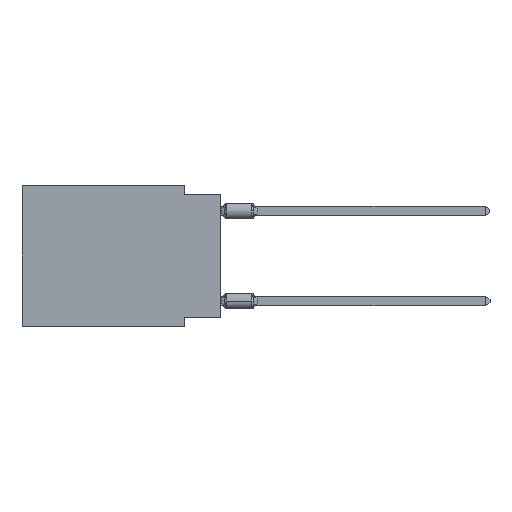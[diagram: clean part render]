
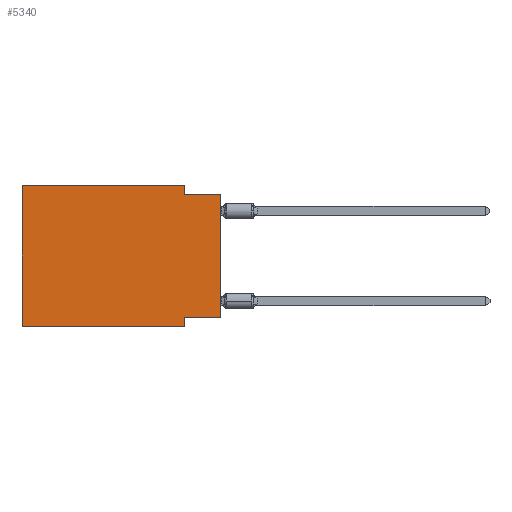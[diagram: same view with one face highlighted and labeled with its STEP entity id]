
A CAD part, left-side view. The second image highlights one B-rep face of the part: STEP entity #5340.
In plain terms, the highlighted planar face has unit normal (-1, 0, 0).
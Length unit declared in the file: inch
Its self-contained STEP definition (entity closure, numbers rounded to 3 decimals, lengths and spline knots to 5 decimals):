
#259 = LINE ( 'NONE', #17648, #6496 ) ;
#445 = EDGE_CURVE ( 'NONE', #4092, #9100, #18536, .T. ) ;
#514 = VERTEX_POINT ( 'NONE', #1994 ) ;
#1445 = EDGE_LOOP ( 'NONE', ( #12700, #13799, #5948, #2349, #14750, #10892, #8039, #2015 ) ) ;
#1649 = CARTESIAN_POINT ( 'NONE',  ( 0., 0.1, -0.025 ) ) ;
#1694 = VECTOR ( 'NONE', #16999, 39.37008 ) ;
#1905 = CARTESIAN_POINT ( 'NONE',  ( 0., 0., -0.365 ) ) ;
#1994 = CARTESIAN_POINT ( 'NONE',  ( 0., 0.1, 0. ) ) ;
#2015 = ORIENTED_EDGE ( 'NONE', *, *, #4276, .F. ) ;
#2109 = CARTESIAN_POINT ( 'NONE',  ( 0., 0.55, -0.39 ) ) ;
#2139 = CARTESIAN_POINT ( 'NONE',  ( 0., 0.55, 0. ) ) ;
#2317 = CARTESIAN_POINT ( 'NONE',  ( 0., 0.55, 0. ) ) ;
#2349 = ORIENTED_EDGE ( 'NONE', *, *, #6846, .F. ) ;
#2357 = CARTESIAN_POINT ( 'NONE',  ( 0., 0.1, -0.365 ) ) ;
#2386 = EDGE_CURVE ( 'NONE', #9490, #3040, #17271, .T. ) ;
#2815 = CARTESIAN_POINT ( 'NONE',  ( 0., 0.55, 0. ) ) ;
#2879 = VECTOR ( 'NONE', #5657, 39.37008 ) ;
#3040 = VERTEX_POINT ( 'NONE', #16275 ) ;
#3069 = DIRECTION ( 'NONE',  ( 0., 0., 1. ) ) ;
#3242 = VECTOR ( 'NONE', #17479, 39.37008 ) ;
#3299 = EDGE_CURVE ( 'NONE', #15365, #9100, #11369, .T. ) ;
#3946 = VERTEX_POINT ( 'NONE', #2317 ) ;
#4092 = VERTEX_POINT ( 'NONE', #18384 ) ;
#4115 = AXIS2_PLACEMENT_3D ( 'NONE', #2139, #12278, #6644 ) ;
#4240 = CARTESIAN_POINT ( 'NONE',  ( 0., 0., -0.025 ) ) ;
#4276 = EDGE_CURVE ( 'NONE', #4092, #9490, #10543, .T. ) ;
#5052 = VECTOR ( 'NONE', #8529, 39.37008 ) ;
#5340 = ADVANCED_FACE ( 'NONE', ( #15003 ), #6553, .F. ) ;
#5619 = CARTESIAN_POINT ( 'NONE',  ( 0., 0.1, -0.39 ) ) ;
#5657 = DIRECTION ( 'NONE',  ( 0., 0., 1. ) ) ;
#5948 = ORIENTED_EDGE ( 'NONE', *, *, #16321, .F. ) ;
#6496 = VECTOR ( 'NONE', #3069, 39.37008 ) ;
#6553 = PLANE ( 'NONE',  #4115 ) ;
#6644 = DIRECTION ( 'NONE',  ( 0., 0., -1. ) ) ;
#6846 = EDGE_CURVE ( 'NONE', #3946, #514, #11359, .T. ) ;
#7033 = EDGE_CURVE ( 'NONE', #7882, #3040, #14924, .T. ) ;
#7528 = VECTOR ( 'NONE', #14961, 39.37008 ) ;
#7882 = VERTEX_POINT ( 'NONE', #2109 ) ;
#8039 = ORIENTED_EDGE ( 'NONE', *, *, #2386, .F. ) ;
#8529 = DIRECTION ( 'NONE',  ( 0., -1., 0. ) ) ;
#9100 = VERTEX_POINT ( 'NONE', #9234 ) ;
#9234 = CARTESIAN_POINT ( 'NONE',  ( 0., 0., -0.025 ) ) ;
#9245 = VECTOR ( 'NONE', #9959, 39.37008 ) ;
#9490 = VERTEX_POINT ( 'NONE', #2357 ) ;
#9830 = DIRECTION ( 'NONE',  ( 0., 0., -1. ) ) ;
#9959 = DIRECTION ( 'NONE',  ( 0., -1., 0. ) ) ;
#10543 = LINE ( 'NONE', #1905, #7528 ) ;
#10892 = ORIENTED_EDGE ( 'NONE', *, *, #7033, .T. ) ;
#11359 = LINE ( 'NONE', #2815, #5052 ) ;
#11369 = LINE ( 'NONE', #4240, #9245 ) ;
#11735 = CARTESIAN_POINT ( 'NONE',  ( 0., 0.55, -0.39 ) ) ;
#12278 = DIRECTION ( 'NONE',  ( 1., 0., 0. ) ) ;
#12700 = ORIENTED_EDGE ( 'NONE', *, *, #445, .T. ) ;
#13799 = ORIENTED_EDGE ( 'NONE', *, *, #3299, .F. ) ;
#14479 = CARTESIAN_POINT ( 'NONE',  ( 0., 0., 0. ) ) ;
#14750 = ORIENTED_EDGE ( 'NONE', *, *, #17656, .F. ) ;
#14924 = LINE ( 'NONE', #11735, #3242 ) ;
#14961 = DIRECTION ( 'NONE',  ( 0., 1., 0. ) ) ;
#15003 = FACE_OUTER_BOUND ( 'NONE', #1445, .T. ) ;
#15365 = VERTEX_POINT ( 'NONE', #1649 ) ;
#16275 = CARTESIAN_POINT ( 'NONE',  ( 0., 0.1, -0.39 ) ) ;
#16321 = EDGE_CURVE ( 'NONE', #514, #15365, #18217, .T. ) ;
#16962 = VECTOR ( 'NONE', #9830, 39.37008 ) ;
#16999 = DIRECTION ( 'NONE',  ( 0., 0., -1. ) ) ;
#17271 = LINE ( 'NONE', #5619, #1694 ) ;
#17479 = DIRECTION ( 'NONE',  ( 0., -1., 0. ) ) ;
#17648 = CARTESIAN_POINT ( 'NONE',  ( 0., 0.55, 0. ) ) ;
#17656 = EDGE_CURVE ( 'NONE', #7882, #3946, #259, .T. ) ;
#18217 = LINE ( 'NONE', #18304, #16962 ) ;
#18304 = CARTESIAN_POINT ( 'NONE',  ( 0., 0.1, 0. ) ) ;
#18384 = CARTESIAN_POINT ( 'NONE',  ( 0., 0., -0.365 ) ) ;
#18536 = LINE ( 'NONE', #14479, #2879 ) ;
